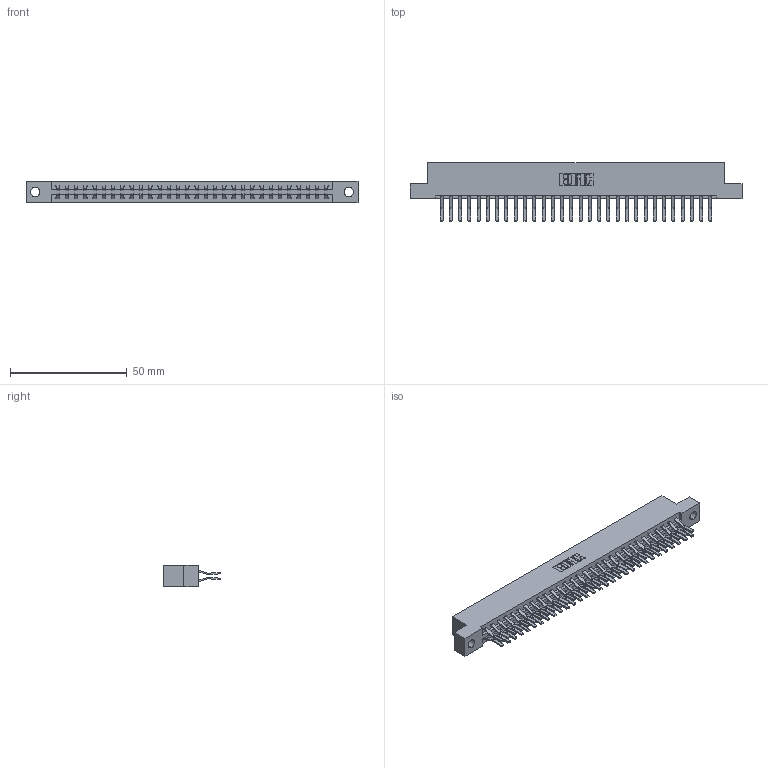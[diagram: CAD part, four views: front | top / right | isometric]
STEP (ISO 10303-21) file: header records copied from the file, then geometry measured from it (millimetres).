
FILE_DESCRIPTION (( 'STEP AP203' ), '1' );
FILE_NAME ('337-060-560-204.STEP', '2018-08-10T09:18:40', ( '' ), ( '' ), 'SwSTEP 2.0', 'SolidWorks 2016', '' );
FILE_SCHEMA (( 'CONFIG_CONTROL_DESIGN' ));
Length unit declared in the file: inch
Products named in the file (3): 337 Part_Flush Mounting Lugs - 0.156 Dia-TH; 345-292-001_560 Tail; 337-060-560-204
Assembly tree (61 placements, depth 2):
  337-060-560-204
    337 Part_Flush Mounting Lugs - 0.156 Dia-TH
    345-292-001_560 Tail  x60
Bounding box: 141.88 x 24.78 x 9.4 mm (x, y, z)
Volume: 15098.6 mm3; surface area: 17888.1 mm2
Topology: 61 solids, 61 shells, 3474 faces, 10331 edges, 6806 vertices
Faces by surface type: plane 2350, cylinder 1124
Entity records: 24903 total; most frequent: CARTESIAN_POINT 4206, ORIENTED_EDGE 4142, DIRECTION 3603, EDGE_CURVE 2071, LINE 1939, VECTOR 1939, VERTEX_POINT 1378, AXIS2_PLACEMENT_3D 832
